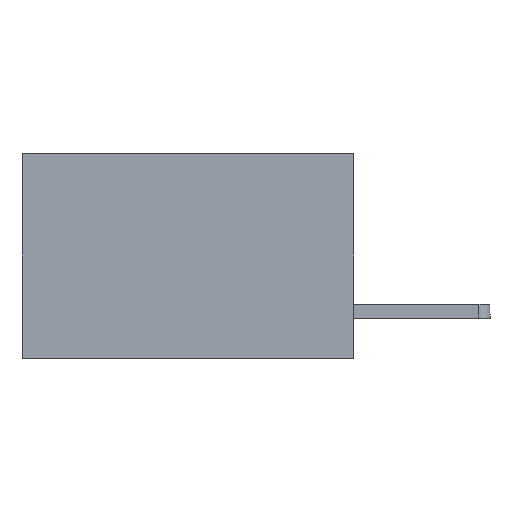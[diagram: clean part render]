
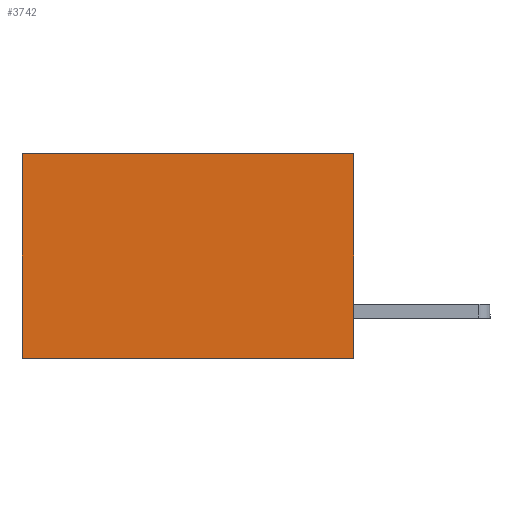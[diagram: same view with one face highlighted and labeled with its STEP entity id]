
A CAD part, left-side view. The second image highlights one B-rep face of the part: STEP entity #3742.
In plain terms, the highlighted planar face has unit normal (-1, 0, 0).
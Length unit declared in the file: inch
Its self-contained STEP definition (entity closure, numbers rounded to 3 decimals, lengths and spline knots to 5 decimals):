
#607 = VERTEX_POINT ( 'NONE', #3813 ) ;
#1602 = CARTESIAN_POINT ( 'NONE',  ( 0.2875, 0., -0.37 ) ) ;
#1791 = AXIS2_PLACEMENT_3D ( 'NONE', #6460, #8819, #8575 ) ;
#2041 = EDGE_CURVE ( 'NONE', #6217, #5995, #2501, .T. ) ;
#2103 = EDGE_CURVE ( 'NONE', #5995, #5737, #9208, .T. ) ;
#2111 = ORIENTED_EDGE ( 'NONE', *, *, #2041, .F. ) ;
#2131 = CARTESIAN_POINT ( 'NONE',  ( 0.2875, 0., 0. ) ) ;
#2501 = LINE ( 'NONE', #5340, #8054 ) ;
#2926 = CARTESIAN_POINT ( 'NONE',  ( 0.2875, 0., 0. ) ) ;
#3350 = EDGE_LOOP ( 'NONE', ( #5580, #4652, #2111, #5727 ) ) ;
#3459 = VECTOR ( 'NONE', #4503, 39.37008 ) ;
#3742 = ADVANCED_FACE ( 'NONE', ( #4988 ), #9394, .F. ) ;
#3813 = CARTESIAN_POINT ( 'NONE',  ( 0.2875, 0.6, 0. ) ) ;
#4503 = DIRECTION ( 'NONE',  ( 0., 0., -1. ) ) ;
#4528 = EDGE_CURVE ( 'NONE', #607, #5737, #5452, .T. ) ;
#4652 = ORIENTED_EDGE ( 'NONE', *, *, #2103, .F. ) ;
#4692 = CARTESIAN_POINT ( 'NONE',  ( 0.2875, 0., -0.37 ) ) ;
#4707 = DIRECTION ( 'NONE',  ( 0., 1., 0. ) ) ;
#4988 = FACE_OUTER_BOUND ( 'NONE', #3350, .T. ) ;
#5064 = VECTOR ( 'NONE', #5748, 39.37008 ) ;
#5125 = DIRECTION ( 'NONE',  ( 0., 0., -1. ) ) ;
#5340 = CARTESIAN_POINT ( 'NONE',  ( 0.2875, 0., 0. ) ) ;
#5452 = LINE ( 'NONE', #7178, #3459 ) ;
#5580 = ORIENTED_EDGE ( 'NONE', *, *, #4528, .T. ) ;
#5727 = ORIENTED_EDGE ( 'NONE', *, *, #6940, .T. ) ;
#5737 = VERTEX_POINT ( 'NONE', #7092 ) ;
#5748 = DIRECTION ( 'NONE',  ( 0., 1., 0. ) ) ;
#5995 = VERTEX_POINT ( 'NONE', #1602 ) ;
#6217 = VERTEX_POINT ( 'NONE', #2926 ) ;
#6460 = CARTESIAN_POINT ( 'NONE',  ( 0.2875, 0., 0. ) ) ;
#6940 = EDGE_CURVE ( 'NONE', #6217, #607, #8820, .T. ) ;
#7092 = CARTESIAN_POINT ( 'NONE',  ( 0.2875, 0.6, -0.37 ) ) ;
#7178 = CARTESIAN_POINT ( 'NONE',  ( 0.2875, 0.6, 0. ) ) ;
#7833 = VECTOR ( 'NONE', #4707, 39.37008 ) ;
#8054 = VECTOR ( 'NONE', #5125, 39.37008 ) ;
#8575 = DIRECTION ( 'NONE',  ( 0., 0., -1. ) ) ;
#8819 = DIRECTION ( 'NONE',  ( 1., 0., 0. ) ) ;
#8820 = LINE ( 'NONE', #2131, #5064 ) ;
#9208 = LINE ( 'NONE', #4692, #7833 ) ;
#9394 = PLANE ( 'NONE',  #1791 ) ;
